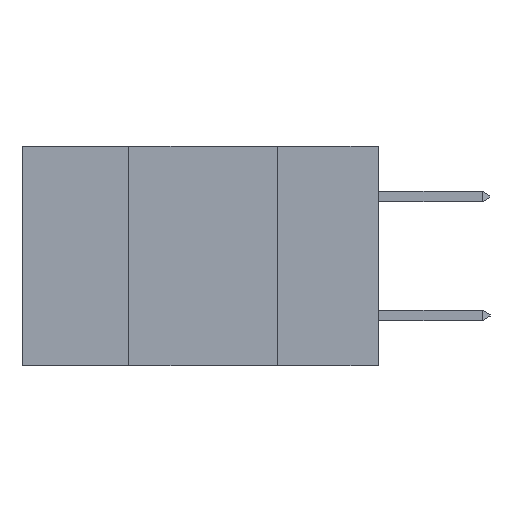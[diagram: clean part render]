
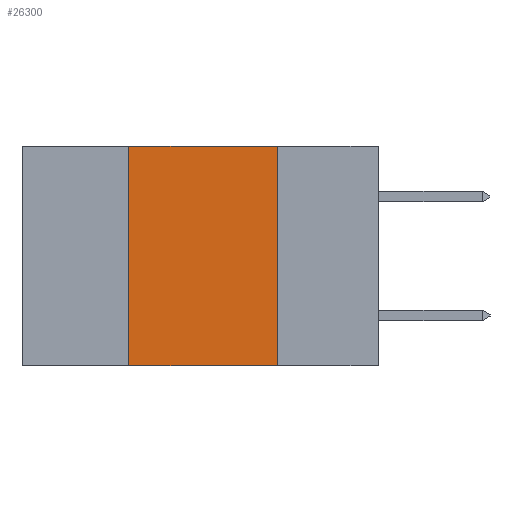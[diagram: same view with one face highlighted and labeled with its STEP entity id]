
A CAD part, left-side view. The second image highlights one B-rep face of the part: STEP entity #26300.
In plain terms, the highlighted planar face has unit normal (-1, 0, 0).
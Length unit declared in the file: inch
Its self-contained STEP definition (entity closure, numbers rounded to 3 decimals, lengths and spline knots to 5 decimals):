
#894 = ORIENTED_EDGE ( 'NONE', *, *, #22004, .T. ) ;
#1680 = CARTESIAN_POINT ( 'NONE',  ( 0., 0.42, -0.37 ) ) ;
#1804 = CARTESIAN_POINT ( 'NONE',  ( 0., 0.42, -0.37 ) ) ;
#2625 = CARTESIAN_POINT ( 'NONE',  ( 0., 0.17, 0. ) ) ;
#2859 = DIRECTION ( 'NONE',  ( 1., 0., 0. ) ) ;
#3676 = CARTESIAN_POINT ( 'NONE',  ( 0., 0.17, -0.37 ) ) ;
#3854 = DIRECTION ( 'NONE',  ( 0., 0., 1. ) ) ;
#4052 = EDGE_CURVE ( 'NONE', #18909, #11731, #7202, .T. ) ;
#4093 = VECTOR ( 'NONE', #14425, 39.37008 ) ;
#5739 = DIRECTION ( 'NONE',  ( 0., 0., -1. ) ) ;
#6998 = VECTOR ( 'NONE', #3854, 39.37008 ) ;
#7202 = LINE ( 'NONE', #26183, #16861 ) ;
#10298 = CARTESIAN_POINT ( 'NONE',  ( 0., 0.6, -0.37 ) ) ;
#10490 = ORIENTED_EDGE ( 'NONE', *, *, #17246, .F. ) ;
#11731 = VERTEX_POINT ( 'NONE', #2625 ) ;
#13105 = LINE ( 'NONE', #1804, #6998 ) ;
#14038 = VECTOR ( 'NONE', #5739, 39.37008 ) ;
#14092 = DIRECTION ( 'NONE',  ( 0., -1., 0. ) ) ;
#14425 = DIRECTION ( 'NONE',  ( 0., -1., 0. ) ) ;
#15151 = CARTESIAN_POINT ( 'NONE',  ( 0., 0.6, 0. ) ) ;
#16861 = VECTOR ( 'NONE', #14092, 39.37008 ) ;
#17220 = DIRECTION ( 'NONE',  ( 0., 0., -1. ) ) ;
#17246 = EDGE_CURVE ( 'NONE', #17946, #18909, #13105, .T. ) ;
#17946 = VERTEX_POINT ( 'NONE', #1680 ) ;
#18797 = ORIENTED_EDGE ( 'NONE', *, *, #21833, .F. ) ;
#18909 = VERTEX_POINT ( 'NONE', #25084 ) ;
#19312 = AXIS2_PLACEMENT_3D ( 'NONE', #15151, #2859, #17220 ) ;
#20399 = LINE ( 'NONE', #10298, #4093 ) ;
#20554 = VERTEX_POINT ( 'NONE', #21808 ) ;
#21190 = PLANE ( 'NONE',  #19312 ) ;
#21808 = CARTESIAN_POINT ( 'NONE',  ( 0., 0.17, -0.37 ) ) ;
#21833 = EDGE_CURVE ( 'NONE', #11731, #20554, #24218, .T. ) ;
#22004 = EDGE_CURVE ( 'NONE', #17946, #20554, #20399, .T. ) ;
#24218 = LINE ( 'NONE', #3676, #14038 ) ;
#24826 = ORIENTED_EDGE ( 'NONE', *, *, #4052, .F. ) ;
#25084 = CARTESIAN_POINT ( 'NONE',  ( 0., 0.42, 0. ) ) ;
#25269 = FACE_OUTER_BOUND ( 'NONE', #25752, .T. ) ;
#25752 = EDGE_LOOP ( 'NONE', ( #18797, #24826, #10490, #894 ) ) ;
#26183 = CARTESIAN_POINT ( 'NONE',  ( 0., 0.6, 0. ) ) ;
#26300 = ADVANCED_FACE ( 'NONE', ( #25269 ), #21190, .F. ) ;
